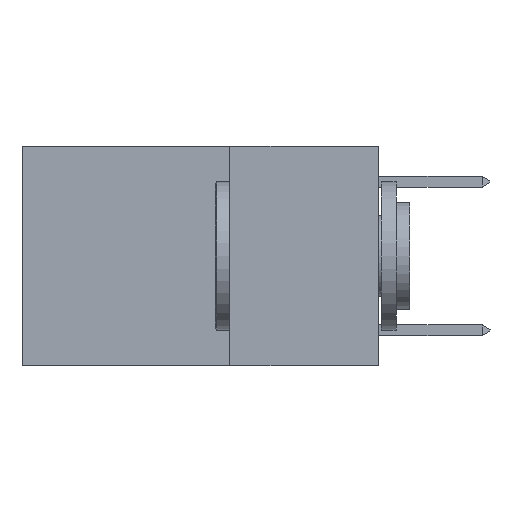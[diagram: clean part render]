
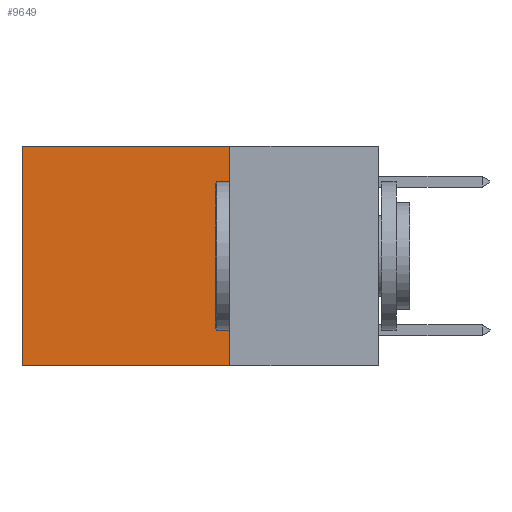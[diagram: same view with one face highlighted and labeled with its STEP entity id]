
A CAD part, left-side view. The second image highlights one B-rep face of the part: STEP entity #9649.
In plain terms, the highlighted planar face has unit normal (-1, 0, 0).
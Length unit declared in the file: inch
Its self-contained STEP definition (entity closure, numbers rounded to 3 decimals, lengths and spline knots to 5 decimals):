
#1371 = DIRECTION ( 'NONE',  ( 0., 0., -1. ) ) ;
#1865 = LINE ( 'NONE', #3302, #17856 ) ;
#2938 = DIRECTION ( 'NONE',  ( 0., 1., 0. ) ) ;
#3302 = CARTESIAN_POINT ( 'NONE',  ( 0.2625, 0.25, 0. ) ) ;
#4142 = ORIENTED_EDGE ( 'NONE', *, *, #17897, .T. ) ;
#4153 = CARTESIAN_POINT ( 'NONE',  ( 0.2625, 0.25, 0. ) ) ;
#4469 = VERTEX_POINT ( 'NONE', #4153 ) ;
#4657 = CARTESIAN_POINT ( 'NONE',  ( 0.2625, 0.25, 0. ) ) ;
#5110 = CARTESIAN_POINT ( 'NONE',  ( 0.2625, 0.25, -0.37 ) ) ;
#6261 = EDGE_LOOP ( 'NONE', ( #9655, #15002, #7431, #4142 ) ) ;
#6373 = EDGE_CURVE ( 'NONE', #10189, #18053, #14386, .T. ) ;
#7431 = ORIENTED_EDGE ( 'NONE', *, *, #13302, .F. ) ;
#7588 = CARTESIAN_POINT ( 'NONE',  ( 0.2625, 0.25, 0. ) ) ;
#7982 = CARTESIAN_POINT ( 'NONE',  ( 0.2625, 0.6, 0. ) ) ;
#9027 = VECTOR ( 'NONE', #13206, 39.37008 ) ;
#9649 = ADVANCED_FACE ( 'NONE', ( #16336 ), #15488, .F. ) ;
#9655 = ORIENTED_EDGE ( 'NONE', *, *, #15471, .T. ) ;
#9805 = DIRECTION ( 'NONE',  ( 0., 0., -1. ) ) ;
#10114 = CARTESIAN_POINT ( 'NONE',  ( 0.2625, 0.6, 0. ) ) ;
#10189 = VERTEX_POINT ( 'NONE', #12893 ) ;
#12893 = CARTESIAN_POINT ( 'NONE',  ( 0.2625, 0.25, -0.37 ) ) ;
#13061 = DIRECTION ( 'NONE',  ( 0., 1., 0. ) ) ;
#13206 = DIRECTION ( 'NONE',  ( 0., 0., -1. ) ) ;
#13302 = EDGE_CURVE ( 'NONE', #4469, #10189, #1865, .T. ) ;
#14386 = LINE ( 'NONE', #5110, #15672 ) ;
#15002 = ORIENTED_EDGE ( 'NONE', *, *, #6373, .F. ) ;
#15306 = LINE ( 'NONE', #7588, #16926 ) ;
#15471 = EDGE_CURVE ( 'NONE', #16096, #18053, #18231, .T. ) ;
#15488 = PLANE ( 'NONE',  #19978 ) ;
#15584 = DIRECTION ( 'NONE',  ( 1., 0., 0. ) ) ;
#15672 = VECTOR ( 'NONE', #13061, 39.37008 ) ;
#16096 = VERTEX_POINT ( 'NONE', #7982 ) ;
#16184 = CARTESIAN_POINT ( 'NONE',  ( 0.2625, 0.6, -0.37 ) ) ;
#16336 = FACE_OUTER_BOUND ( 'NONE', #6261, .T. ) ;
#16926 = VECTOR ( 'NONE', #2938, 39.37008 ) ;
#17856 = VECTOR ( 'NONE', #9805, 39.37008 ) ;
#17897 = EDGE_CURVE ( 'NONE', #4469, #16096, #15306, .T. ) ;
#18053 = VERTEX_POINT ( 'NONE', #16184 ) ;
#18231 = LINE ( 'NONE', #10114, #9027 ) ;
#19978 = AXIS2_PLACEMENT_3D ( 'NONE', #4657, #15584, #1371 ) ;
